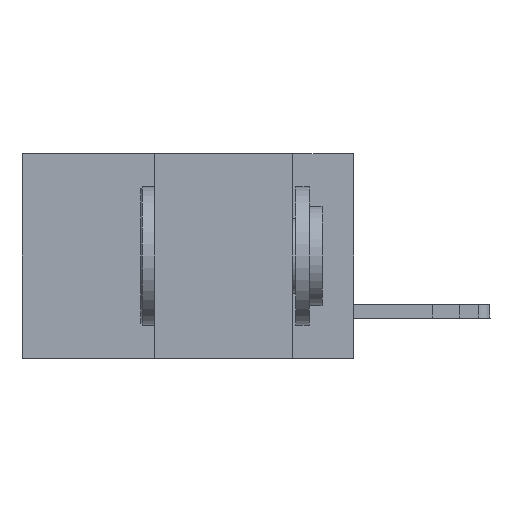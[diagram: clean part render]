
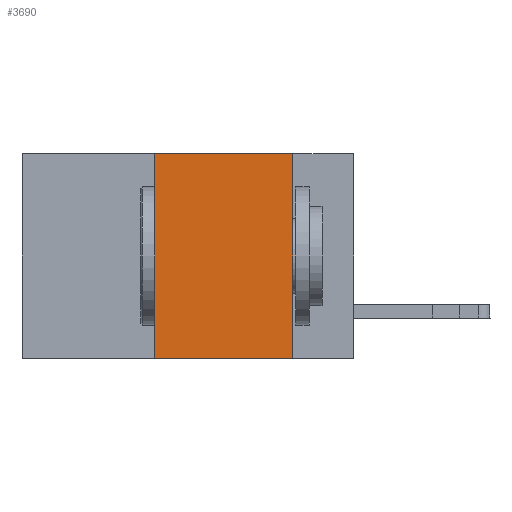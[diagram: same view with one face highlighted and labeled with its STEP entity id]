
A CAD part, left-side view. The second image highlights one B-rep face of the part: STEP entity #3690.
In plain terms, the highlighted planar face has unit normal (-1, 0, 0).
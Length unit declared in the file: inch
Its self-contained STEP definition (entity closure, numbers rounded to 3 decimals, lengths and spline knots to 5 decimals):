
#378 = VECTOR ( 'NONE', #5997, 39.37008 ) ;
#1724 = ORIENTED_EDGE ( 'NONE', *, *, #5838, .F. ) ;
#2114 = CARTESIAN_POINT ( 'NONE',  ( 0., 0.11, 0. ) ) ;
#2628 = VERTEX_POINT ( 'NONE', #15274 ) ;
#2875 = VECTOR ( 'NONE', #17015, 39.37008 ) ;
#3690 = ADVANCED_FACE ( 'NONE', ( #19078 ), #16942, .F. ) ;
#3959 = DIRECTION ( 'NONE',  ( 0., -1., 0. ) ) ;
#3998 = CARTESIAN_POINT ( 'NONE',  ( 0., 0.11, -0.37 ) ) ;
#5402 = VERTEX_POINT ( 'NONE', #3998 ) ;
#5838 = EDGE_CURVE ( 'NONE', #6412, #13760, #16719, .T. ) ;
#5843 = VECTOR ( 'NONE', #29818, 39.37008 ) ;
#5997 = DIRECTION ( 'NONE',  ( 0., 0., 1. ) ) ;
#6412 = VERTEX_POINT ( 'NONE', #25099 ) ;
#6886 = LINE ( 'NONE', #2114, #2875 ) ;
#6928 = CARTESIAN_POINT ( 'NONE',  ( 0., 0.6, -0.37 ) ) ;
#7392 = ORIENTED_EDGE ( 'NONE', *, *, #7802, .F. ) ;
#7419 = ORIENTED_EDGE ( 'NONE', *, *, #30776, .T. ) ;
#7802 = EDGE_CURVE ( 'NONE', #2628, #6412, #8468, .T. ) ;
#8385 = CARTESIAN_POINT ( 'NONE',  ( 0., 0.11, 0. ) ) ;
#8468 = LINE ( 'NONE', #28257, #378 ) ;
#8612 = VECTOR ( 'NONE', #3959, 39.37008 ) ;
#8905 = ORIENTED_EDGE ( 'NONE', *, *, #19061, .F. ) ;
#13760 = VERTEX_POINT ( 'NONE', #8385 ) ;
#15274 = CARTESIAN_POINT ( 'NONE',  ( 0., 0.36, -0.37 ) ) ;
#16719 = LINE ( 'NONE', #16876, #8612 ) ;
#16876 = CARTESIAN_POINT ( 'NONE',  ( 0., 0.6, 0. ) ) ;
#16942 = PLANE ( 'NONE',  #20076 ) ;
#17015 = DIRECTION ( 'NONE',  ( 0., 0., -1. ) ) ;
#19061 = EDGE_CURVE ( 'NONE', #13760, #5402, #6886, .T. ) ;
#19078 = FACE_OUTER_BOUND ( 'NONE', #20401, .T. ) ;
#20076 = AXIS2_PLACEMENT_3D ( 'NONE', #29390, #31684, #23805 ) ;
#20401 = EDGE_LOOP ( 'NONE', ( #8905, #1724, #7392, #7419 ) ) ;
#23805 = DIRECTION ( 'NONE',  ( 0., 0., -1. ) ) ;
#25099 = CARTESIAN_POINT ( 'NONE',  ( 0., 0.36, 0. ) ) ;
#28257 = CARTESIAN_POINT ( 'NONE',  ( 0., 0.36, 0. ) ) ;
#29390 = CARTESIAN_POINT ( 'NONE',  ( 0., 0.6, 0. ) ) ;
#29818 = DIRECTION ( 'NONE',  ( 0., -1., 0. ) ) ;
#29974 = LINE ( 'NONE', #6928, #5843 ) ;
#30776 = EDGE_CURVE ( 'NONE', #2628, #5402, #29974, .T. ) ;
#31684 = DIRECTION ( 'NONE',  ( 1., 0., 0. ) ) ;
